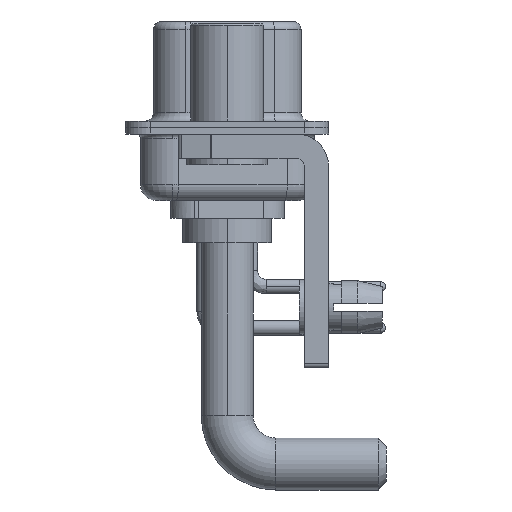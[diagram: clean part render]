
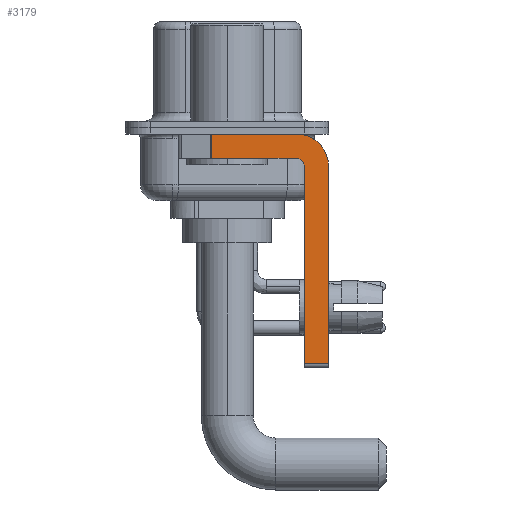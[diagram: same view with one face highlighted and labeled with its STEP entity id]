
A CAD part, left-side view. The second image highlights one B-rep face of the part: STEP entity #3179.
In plain terms, the highlighted planar face has unit normal (-1, 0, 0).
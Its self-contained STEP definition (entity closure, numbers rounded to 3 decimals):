
#92 = EDGE_CURVE ( 'NONE', #1646, #21321, #17081, .T. ) ;
#177 = CARTESIAN_POINT ( 'NONE',  ( -2.9, -4.25, -2.4 ) ) ;
#810 = AXIS2_PLACEMENT_3D ( 'NONE', #817, #22487, #9438 ) ;
#817 = CARTESIAN_POINT ( 'NONE',  ( -2.9, -4.25, -2.4 ) ) ;
#896 = CARTESIAN_POINT ( 'NONE',  ( -2.9, 0.978, -0.4 ) ) ;
#1065 = CARTESIAN_POINT ( 'NONE',  ( -2.9, 0.978, -1.9 ) ) ;
#1420 = CARTESIAN_POINT ( 'NONE',  ( -2.9, -6.25, -2.4 ) ) ;
#1617 = CARTESIAN_POINT ( 'NONE',  ( -2.9, -4.75, -14.8 ) ) ;
#1646 = VERTEX_POINT ( 'NONE', #16047 ) ;
#2436 = VECTOR ( 'NONE', #24331, 1000. ) ;
#3179 = ADVANCED_FACE ( 'NONE', ( #26256 ), #21700, .F. ) ;
#3786 = EDGE_CURVE ( 'NONE', #24416, #7486, #10278, .T. ) ;
#4984 = AXIS2_PLACEMENT_3D ( 'NONE', #17839, #13571, #17976 ) ;
#5049 = VECTOR ( 'NONE', #20781, 1000. ) ;
#5680 = DIRECTION ( 'NONE',  ( 0., -1., 0. ) ) ;
#6345 = EDGE_CURVE ( 'NONE', #7529, #21321, #9143, .T. ) ;
#6714 = ORIENTED_EDGE ( 'NONE', *, *, #15764, .F. ) ;
#7486 = VERTEX_POINT ( 'NONE', #27121 ) ;
#7529 = VERTEX_POINT ( 'NONE', #896 ) ;
#7703 = ORIENTED_EDGE ( 'NONE', *, *, #18399, .F. ) ;
#8121 = LINE ( 'NONE', #1617, #16061 ) ;
#8305 = ORIENTED_EDGE ( 'NONE', *, *, #3786, .T. ) ;
#8443 = CARTESIAN_POINT ( 'NONE',  ( -2.9, -4.75, -14.55 ) ) ;
#8488 = ORIENTED_EDGE ( 'NONE', *, *, #10603, .F. ) ;
#8624 = EDGE_CURVE ( 'NONE', #9367, #7486, #13071, .T. ) ;
#8701 = DIRECTION ( 'NONE',  ( 0., 1., 0. ) ) ;
#9143 = LINE ( 'NONE', #26473, #2436 ) ;
#9367 = VERTEX_POINT ( 'NONE', #1420 ) ;
#9438 = DIRECTION ( 'NONE',  ( 0., 0., -1. ) ) ;
#9969 = CARTESIAN_POINT ( 'NONE',  ( -2.9, -4.75, -2.4 ) ) ;
#10278 = LINE ( 'NONE', #27322, #5049 ) ;
#10349 = ORIENTED_EDGE ( 'NONE', *, *, #26979, .F. ) ;
#10603 = EDGE_CURVE ( 'NONE', #19447, #1646, #20808, .T. ) ;
#10729 = VECTOR ( 'NONE', #5680, 1000. ) ;
#10783 = DIRECTION ( 'NONE',  ( 1., 0., 0. ) ) ;
#11324 = ORIENTED_EDGE ( 'NONE', *, *, #92, .F. ) ;
#13071 = LINE ( 'NONE', #19751, #17759 ) ;
#13375 = CARTESIAN_POINT ( 'NONE',  ( -2.9, -4.25, -1.9 ) ) ;
#13571 = DIRECTION ( 'NONE',  ( -1., 0., 0. ) ) ;
#14495 = DIRECTION ( 'NONE',  ( 0., 0., 1. ) ) ;
#15069 = AXIS2_PLACEMENT_3D ( 'NONE', #177, #10783, #21415 ) ;
#15764 = EDGE_CURVE ( 'NONE', #24416, #19447, #8121, .T. ) ;
#15856 = VERTEX_POINT ( 'NONE', #25421 ) ;
#16047 = CARTESIAN_POINT ( 'NONE',  ( -2.9, -4.25, -1.9 ) ) ;
#16061 = VECTOR ( 'NONE', #14495, 1000. ) ;
#17081 = LINE ( 'NONE', #13375, #20818 ) ;
#17759 = VECTOR ( 'NONE', #19464, 1000. ) ;
#17839 = CARTESIAN_POINT ( 'NONE',  ( -2.9, -4.25, -2.4 ) ) ;
#17976 = DIRECTION ( 'NONE',  ( 0., 0., 1. ) ) ;
#18148 = LINE ( 'NONE', #22404, #10729 ) ;
#18399 = EDGE_CURVE ( 'NONE', #7529, #15856, #18148, .T. ) ;
#19447 = VERTEX_POINT ( 'NONE', #9969 ) ;
#19464 = DIRECTION ( 'NONE',  ( 0., 0., -1. ) ) ;
#19751 = CARTESIAN_POINT ( 'NONE',  ( -2.9, -6.25, -2.4 ) ) ;
#20781 = DIRECTION ( 'NONE',  ( 0., -1., 0. ) ) ;
#20808 = CIRCLE ( 'NONE', #4984, 0.5 ) ;
#20818 = VECTOR ( 'NONE', #8701, 1000. ) ;
#21321 = VERTEX_POINT ( 'NONE', #1065 ) ;
#21415 = DIRECTION ( 'NONE',  ( 0., 0., -1. ) ) ;
#21700 = PLANE ( 'NONE',  #15069 ) ;
#22404 = CARTESIAN_POINT ( 'NONE',  ( -2.9, 3., -0.4 ) ) ;
#22487 = DIRECTION ( 'NONE',  ( 1., 0., 0. ) ) ;
#24331 = DIRECTION ( 'NONE',  ( 0., 0., -1. ) ) ;
#24343 = ORIENTED_EDGE ( 'NONE', *, *, #6345, .T. ) ;
#24416 = VERTEX_POINT ( 'NONE', #8443 ) ;
#25249 = CIRCLE ( 'NONE', #810, 2. ) ;
#25421 = CARTESIAN_POINT ( 'NONE',  ( -2.9, -4.25, -0.4 ) ) ;
#25695 = EDGE_LOOP ( 'NONE', ( #7703, #24343, #11324, #8488, #6714, #8305, #26202, #10349 ) ) ;
#26202 = ORIENTED_EDGE ( 'NONE', *, *, #8624, .F. ) ;
#26256 = FACE_OUTER_BOUND ( 'NONE', #25695, .T. ) ;
#26473 = CARTESIAN_POINT ( 'NONE',  ( -2.9, 0.978, -1.9 ) ) ;
#26979 = EDGE_CURVE ( 'NONE', #15856, #9367, #25249, .T. ) ;
#27121 = CARTESIAN_POINT ( 'NONE',  ( -2.9, -6.25, -14.55 ) ) ;
#27322 = CARTESIAN_POINT ( 'NONE',  ( -2.9, -4.25, -14.55 ) ) ;
